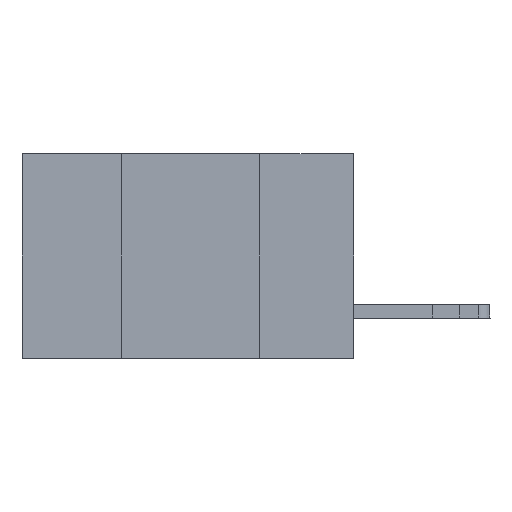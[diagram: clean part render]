
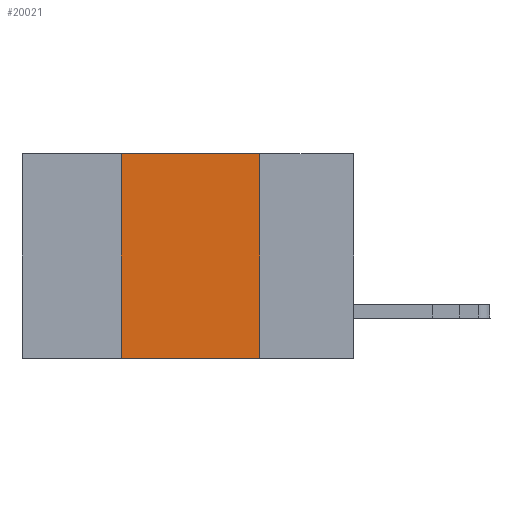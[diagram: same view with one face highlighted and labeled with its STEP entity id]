
A CAD part, left-side view. The second image highlights one B-rep face of the part: STEP entity #20021.
In plain terms, the highlighted planar face has unit normal (-1, 0, 0).
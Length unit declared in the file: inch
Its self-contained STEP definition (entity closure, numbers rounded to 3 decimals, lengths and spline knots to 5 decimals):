
#2210 = VECTOR ( 'NONE', #35769, 39.37008 ) ;
#3938 = VERTEX_POINT ( 'NONE', #35319 ) ;
#5410 = DIRECTION ( 'NONE',  ( 0., -1., 0. ) ) ;
#6635 = VERTEX_POINT ( 'NONE', #11547 ) ;
#7351 = PLANE ( 'NONE',  #23234 ) ;
#8390 = CARTESIAN_POINT ( 'NONE',  ( 0., 0.17, 0. ) ) ;
#8481 = VECTOR ( 'NONE', #23117, 39.37008 ) ;
#10258 = DIRECTION ( 'NONE',  ( 1., 0., 0. ) ) ;
#10674 = ORIENTED_EDGE ( 'NONE', *, *, #17782, .F. ) ;
#11547 = CARTESIAN_POINT ( 'NONE',  ( 0., 0.17, -0.37 ) ) ;
#11880 = EDGE_CURVE ( 'NONE', #15601, #6635, #18138, .T. ) ;
#13420 = ORIENTED_EDGE ( 'NONE', *, *, #11880, .T. ) ;
#15601 = VERTEX_POINT ( 'NONE', #31506 ) ;
#16261 = LINE ( 'NONE', #34669, #8481 ) ;
#16895 = LINE ( 'NONE', #21271, #2210 ) ;
#17644 = EDGE_LOOP ( 'NONE', ( #19304, #24900, #10674, #13420 ) ) ;
#17782 = EDGE_CURVE ( 'NONE', #15601, #3938, #16261, .T. ) ;
#18138 = LINE ( 'NONE', #25946, #28650 ) ;
#18977 = CARTESIAN_POINT ( 'NONE',  ( 0., 0.6, 0. ) ) ;
#19304 = ORIENTED_EDGE ( 'NONE', *, *, #28796, .F. ) ;
#19642 = DIRECTION ( 'NONE',  ( 0., -1., 0. ) ) ;
#20021 = ADVANCED_FACE ( 'NONE', ( #20389 ), #7351, .F. ) ;
#20389 = FACE_OUTER_BOUND ( 'NONE', #17644, .T. ) ;
#21271 = CARTESIAN_POINT ( 'NONE',  ( 0., 0.17, 0. ) ) ;
#23117 = DIRECTION ( 'NONE',  ( 0., 0., 1. ) ) ;
#23234 = AXIS2_PLACEMENT_3D ( 'NONE', #18977, #10258, #30696 ) ;
#24900 = ORIENTED_EDGE ( 'NONE', *, *, #37235, .F. ) ;
#25946 = CARTESIAN_POINT ( 'NONE',  ( 0., 0.6, -0.37 ) ) ;
#27021 = VECTOR ( 'NONE', #19642, 39.37008 ) ;
#28329 = CARTESIAN_POINT ( 'NONE',  ( 0., 0.6, 0. ) ) ;
#28650 = VECTOR ( 'NONE', #5410, 39.37008 ) ;
#28796 = EDGE_CURVE ( 'NONE', #29550, #6635, #16895, .T. ) ;
#29550 = VERTEX_POINT ( 'NONE', #8390 ) ;
#30696 = DIRECTION ( 'NONE',  ( 0., 0., -1. ) ) ;
#31506 = CARTESIAN_POINT ( 'NONE',  ( 0., 0.42, -0.37 ) ) ;
#34669 = CARTESIAN_POINT ( 'NONE',  ( 0., 0.42, 0. ) ) ;
#34708 = LINE ( 'NONE', #28329, #27021 ) ;
#35319 = CARTESIAN_POINT ( 'NONE',  ( 0., 0.42, 0. ) ) ;
#35769 = DIRECTION ( 'NONE',  ( 0., 0., -1. ) ) ;
#37235 = EDGE_CURVE ( 'NONE', #3938, #29550, #34708, .T. ) ;
